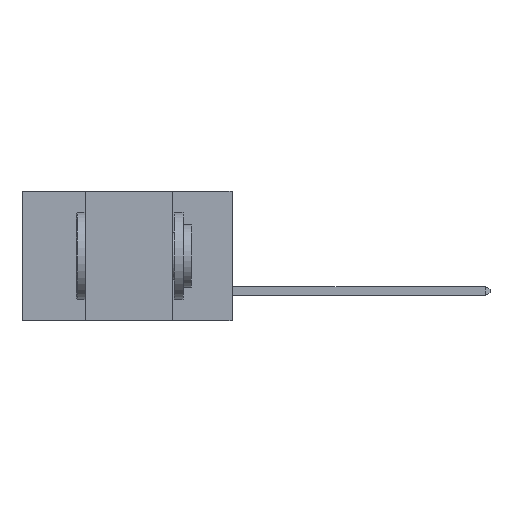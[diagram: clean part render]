
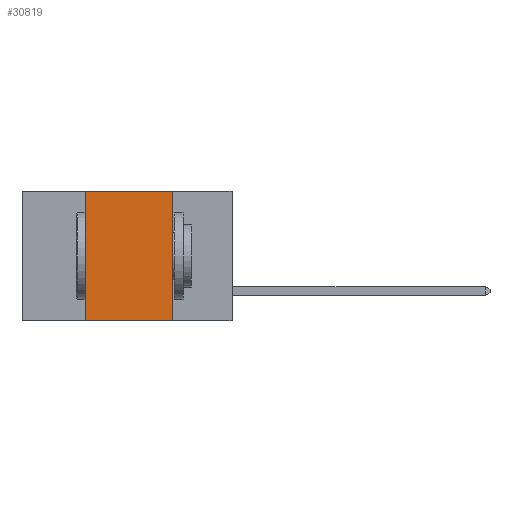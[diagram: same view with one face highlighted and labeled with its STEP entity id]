
A CAD part, left-side view. The second image highlights one B-rep face of the part: STEP entity #30819.
In plain terms, the highlighted planar face has unit normal (-1, 0, 0).
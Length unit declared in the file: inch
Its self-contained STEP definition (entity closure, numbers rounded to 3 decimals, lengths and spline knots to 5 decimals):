
#3381 = LINE ( 'NONE', #33196, #17788 ) ;
#4791 = ORIENTED_EDGE ( 'NONE', *, *, #33225, .F. ) ;
#5457 = CARTESIAN_POINT ( 'NONE',  ( 0., 0.42, 0. ) ) ;
#5529 = VERTEX_POINT ( 'NONE', #6737 ) ;
#5988 = VECTOR ( 'NONE', #10557, 39.37008 ) ;
#6192 = CARTESIAN_POINT ( 'NONE',  ( 0., 0.6, 0. ) ) ;
#6632 = CARTESIAN_POINT ( 'NONE',  ( 0., 0.6, 0. ) ) ;
#6737 = CARTESIAN_POINT ( 'NONE',  ( 0., 0.42, -0.37 ) ) ;
#7266 = ORIENTED_EDGE ( 'NONE', *, *, #22682, .F. ) ;
#9075 = DIRECTION ( 'NONE',  ( 0., -1., 0. ) ) ;
#9497 = VECTOR ( 'NONE', #9075, 39.37008 ) ;
#9515 = DIRECTION ( 'NONE',  ( 0., 0., -1. ) ) ;
#10557 = DIRECTION ( 'NONE',  ( 0., 0., -1. ) ) ;
#12225 = CARTESIAN_POINT ( 'NONE',  ( 0., 0.17, -0.37 ) ) ;
#12705 = VERTEX_POINT ( 'NONE', #5457 ) ;
#13369 = DIRECTION ( 'NONE',  ( 0., 0., 1. ) ) ;
#13603 = FACE_OUTER_BOUND ( 'NONE', #24462, .T. ) ;
#16138 = DIRECTION ( 'NONE',  ( 0., -1., 0. ) ) ;
#17788 = VECTOR ( 'NONE', #16138, 39.37008 ) ;
#18047 = LINE ( 'NONE', #6192, #9497 ) ;
#18056 = VERTEX_POINT ( 'NONE', #12225 ) ;
#18751 = VECTOR ( 'NONE', #13369, 39.37008 ) ;
#20642 = ORIENTED_EDGE ( 'NONE', *, *, #21138, .T. ) ;
#20912 = PLANE ( 'NONE',  #26946 ) ;
#21138 = EDGE_CURVE ( 'NONE', #5529, #18056, #3381, .T. ) ;
#21936 = CARTESIAN_POINT ( 'NONE',  ( 0., 0.17, 0. ) ) ;
#22682 = EDGE_CURVE ( 'NONE', #33917, #18056, #28756, .T. ) ;
#24462 = EDGE_LOOP ( 'NONE', ( #7266, #33702, #4791, #20642 ) ) ;
#24684 = CARTESIAN_POINT ( 'NONE',  ( 0., 0.42, 0. ) ) ;
#25019 = CARTESIAN_POINT ( 'NONE',  ( 0., 0.17, 0. ) ) ;
#26275 = LINE ( 'NONE', #24684, #18751 ) ;
#26603 = DIRECTION ( 'NONE',  ( 1., 0., 0. ) ) ;
#26946 = AXIS2_PLACEMENT_3D ( 'NONE', #6632, #26603, #9515 ) ;
#28756 = LINE ( 'NONE', #21936, #5988 ) ;
#30033 = EDGE_CURVE ( 'NONE', #12705, #33917, #18047, .T. ) ;
#30819 = ADVANCED_FACE ( 'NONE', ( #13603 ), #20912, .F. ) ;
#33196 = CARTESIAN_POINT ( 'NONE',  ( 0., 0.6, -0.37 ) ) ;
#33225 = EDGE_CURVE ( 'NONE', #5529, #12705, #26275, .T. ) ;
#33702 = ORIENTED_EDGE ( 'NONE', *, *, #30033, .F. ) ;
#33917 = VERTEX_POINT ( 'NONE', #25019 ) ;
